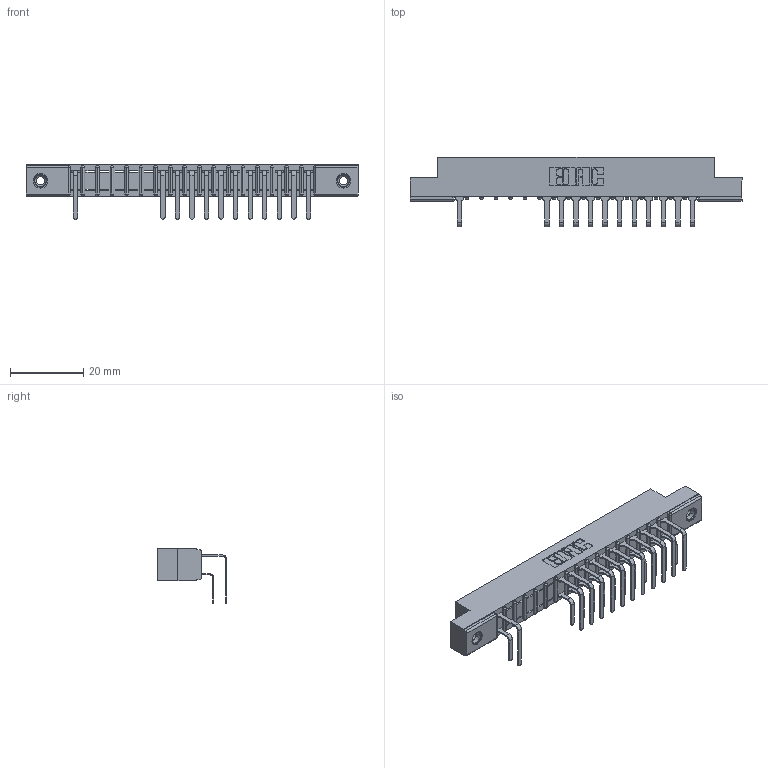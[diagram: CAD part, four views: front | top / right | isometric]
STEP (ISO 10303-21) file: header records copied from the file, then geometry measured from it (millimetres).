
FILE_DESCRIPTION (( 'STEP AP203' ), '1' );
FILE_NAME ('357-017-558-108.STEP', '2018-08-08T03:42:40', ( '' ), ( '' ), 'SwSTEP 2.0', 'SolidWorks 2016', '' );
FILE_SCHEMA (( 'CONFIG_CONTROL_DESIGN' ));
Length unit declared in the file: inch
Products named in the file (5): 307-290-001_558 - 2 (Single); 345-250-001_345-250-003-102; 357-017-558-108; 307 Part_.156 Dia Mounting Holes; 307-290-001_558 559 - 1 (Single)
Assembly tree (27 placements, depth 2):
  357-017-558-108
    307 Part_.156 Dia Mounting Holes
    307-290-001_558 559 - 1 (Single)  x12
    307-290-001_558 - 2 (Single)  x12
    345-250-001_345-250-003-102  x2
Bounding box: 90.37 x 18.96 x 14.81 mm (x, y, z)
Volume: 5882.3 mm3; surface area: 9984.9 mm2
Topology: 27 solids, 27 shells, 1496 faces, 4187 edges, 2702 vertices
Faces by surface type: plane 954, cylinder 490, sphere 36, cone 12, torus 4
Entity records: 20512 total; most frequent: CARTESIAN_POINT 3392, ORIENTED_EDGE 3362, DIRECTION 3331, EDGE_CURVE 1681, LINE 1277, VECTOR 1277, VERTEX_POINT 1088, AXIS2_PLACEMENT_3D 1027
